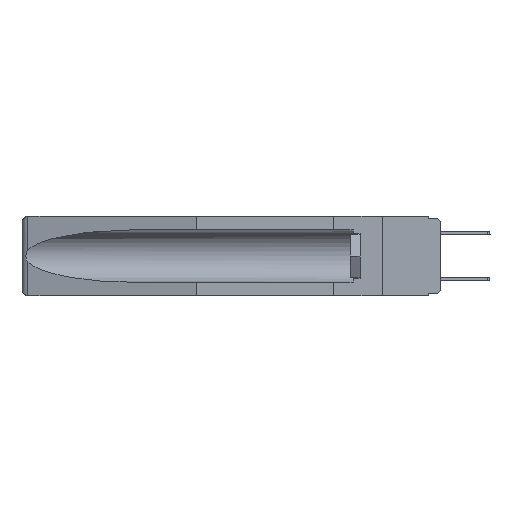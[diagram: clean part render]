
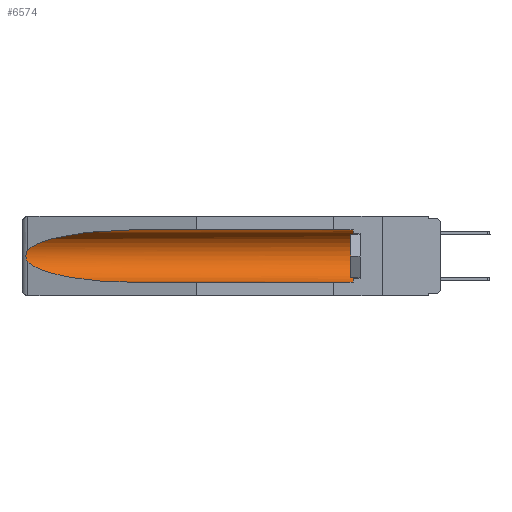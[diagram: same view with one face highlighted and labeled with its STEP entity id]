
A CAD part, left-side view. The second image highlights one B-rep face of the part: STEP entity #6574.
In plain terms, the highlighted cylindrical face has radius 2.857 mm (diameter 5.715 mm), a partial arc.
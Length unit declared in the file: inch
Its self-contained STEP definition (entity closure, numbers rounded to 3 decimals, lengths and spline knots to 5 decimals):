
#9 = CARTESIAN_POINT ( 'NONE',  ( 0.2675, 1.53308, -0.17534 ) ) ;
#93 =( BOUNDED_CURVE ( )  B_SPLINE_CURVE ( 3, ( #5002, #11136, #8118, #14259 ),
 .UNSPECIFIED., .F., .F. ) 
 B_SPLINE_CURVE_WITH_KNOTS ( ( 4, 4 ),
 ( 0.1948, 1.5708 ),
 .UNSPECIFIED. ) 
 CURVE ( )  GEOMETRIC_REPRESENTATION_ITEM ( )  RATIONAL_B_SPLINE_CURVE ( ( 1., 0.848, 0.848, 1. ) ) 
 REPRESENTATION_ITEM ( '' )  );
#108 = FACE_OUTER_BOUND ( 'NONE', #941, .T. ) ;
#810 = CARTESIAN_POINT ( 'NONE',  ( 0.26537, 1.52718, -0.14972 ) ) ;
#941 = EDGE_LOOP ( 'NONE', ( #19492, #7121, #16812, #2679, #1300, #1468 ) ) ;
#1225 = CARTESIAN_POINT ( 'NONE',  ( 0.26597, 1.52961, -0.15275 ) ) ;
#1300 = ORIENTED_EDGE ( 'NONE', *, *, #8733, .T. ) ;
#1468 = ORIENTED_EDGE ( 'NONE', *, *, #6871, .T. ) ;
#1628 = CARTESIAN_POINT ( 'NONE',  ( 0.26537, 1.52718, -0.14972 ) ) ;
#1767 = VERTEX_POINT ( 'NONE', #19756 ) ;
#2050 = CARTESIAN_POINT ( 'NONE',  ( 0.155, 0.126, -0.284 ) ) ;
#2679 = ORIENTED_EDGE ( 'NONE', *, *, #15390, .F. ) ;
#2933 = CARTESIAN_POINT ( 'NONE',  ( 0.26597, 1.5296, -0.19026 ) ) ;
#3026 = LINE ( 'NONE', #10571, #8775 ) ;
#3757 = CARTESIAN_POINT ( 'NONE',  ( 0.26537, 1.52718, -0.19328 ) ) ;
#3776 = AXIS2_PLACEMENT_3D ( 'NONE', #12192, #8975, #9161 ) ;
#4337 = CARTESIAN_POINT ( 'NONE',  ( 0.26537, 1.52718, -0.19328 ) ) ;
#4497 = DIRECTION ( 'NONE',  ( 0., 0., 1. ) ) ;
#5002 = CARTESIAN_POINT ( 'NONE',  ( 0.26537, 1.52718, -0.19328 ) ) ;
#5300 = EDGE_CURVE ( 'NONE', #17446, #18769, #6170, .T. ) ;
#5739 = AXIS2_PLACEMENT_3D ( 'NONE', #15371, #19775, #4497 ) ;
#6170 = B_SPLINE_CURVE_WITH_KNOTS ( 'NONE', 3,
 ( #1628, #1225, #10573, #18117, #19816, #9, #12291, #7372, #2933, #4337 ),
 .UNSPECIFIED., .F., .F.,
 ( 4, 2, 2, 2, 4 ),
 ( 0., 0.00029, 0.00058, 0.00087, 0.00117 ),
 .UNSPECIFIED. ) ;
#6574 = ADVANCED_FACE ( 'NONE', ( #108 ), #7859, .F. ) ;
#6871 = EDGE_CURVE ( 'NONE', #15940, #9825, #19199, .T. ) ;
#6949 = DIRECTION ( 'NONE',  ( 0., 1., 0. ) ) ;
#7121 = ORIENTED_EDGE ( 'NONE', *, *, #5300, .T. ) ;
#7372 = CARTESIAN_POINT ( 'NONE',  ( 0.26655, 1.53094, -0.18657 ) ) ;
#7859 = CYLINDRICAL_SURFACE ( 'NONE', #3776, 0.1125 ) ;
#8118 = CARTESIAN_POINT ( 'NONE',  ( 0.21114, 1.30732, -0.284 ) ) ;
#8733 = EDGE_CURVE ( 'NONE', #12511, #15940, #9894, .T. ) ;
#8775 = VECTOR ( 'NONE', #8867, 39.37008 ) ;
#8867 = DIRECTION ( 'NONE',  ( 0., 1., 0. ) ) ;
#8975 = DIRECTION ( 'NONE',  ( 0., 1., 0. ) ) ;
#9161 = DIRECTION ( 'NONE',  ( 0., 0., 1. ) ) ;
#9825 = VERTEX_POINT ( 'NONE', #13916 ) ;
#9894 = CIRCLE ( 'NONE', #5739, 0.1125 ) ;
#10571 = CARTESIAN_POINT ( 'NONE',  ( 0.155, -0.30754, -0.284 ) ) ;
#10573 = CARTESIAN_POINT ( 'NONE',  ( 0.26654, 1.53092, -0.15636 ) ) ;
#11136 = CARTESIAN_POINT ( 'NONE',  ( 0.25451, 1.48313, -0.24835 ) ) ;
#11821 = VECTOR ( 'NONE', #6949, 39.37008 ) ;
#12000 = EDGE_CURVE ( 'NONE', #18769, #1767, #93, .T. ) ;
#12192 = CARTESIAN_POINT ( 'NONE',  ( 0.155, -0.30754, -0.1715 ) ) ;
#12291 = CARTESIAN_POINT ( 'NONE',  ( 0.2673, 1.53269, -0.17917 ) ) ;
#12511 = VERTEX_POINT ( 'NONE', #2050 ) ;
#12665 = CARTESIAN_POINT ( 'NONE',  ( 0.155, 0.126, -0.059 ) ) ;
#13099 = EDGE_CURVE ( 'NONE', #9825, #17446, #15804, .T. ) ;
#13573 = CARTESIAN_POINT ( 'NONE',  ( 0.26537, 1.52718, -0.14972 ) ) ;
#13768 = CARTESIAN_POINT ( 'NONE',  ( 0.25451, 1.48313, -0.09465 ) ) ;
#13916 = CARTESIAN_POINT ( 'NONE',  ( 0.155, 1.07973, -0.059 ) ) ;
#14259 = CARTESIAN_POINT ( 'NONE',  ( 0.155, 1.07973, -0.284 ) ) ;
#14980 = CARTESIAN_POINT ( 'NONE',  ( 0.155, 1.07973, -0.059 ) ) ;
#15371 = CARTESIAN_POINT ( 'NONE',  ( 0.155, 0.126, -0.1715 ) ) ;
#15390 = EDGE_CURVE ( 'NONE', #12511, #1767, #3026, .T. ) ;
#15804 =( BOUNDED_CURVE ( )  B_SPLINE_CURVE ( 3, ( #14980, #16575, #13768, #13573 ),
 .UNSPECIFIED., .F., .F. ) 
 B_SPLINE_CURVE_WITH_KNOTS ( ( 4, 4 ),
 ( 4.71239, 6.08839 ),
 .UNSPECIFIED. ) 
 CURVE ( )  GEOMETRIC_REPRESENTATION_ITEM ( )  RATIONAL_B_SPLINE_CURVE ( ( 1., 0.848, 0.848, 1. ) ) 
 REPRESENTATION_ITEM ( '' )  );
#15940 = VERTEX_POINT ( 'NONE', #12665 ) ;
#16103 = CARTESIAN_POINT ( 'NONE',  ( 0.155, -0.30754, -0.059 ) ) ;
#16575 = CARTESIAN_POINT ( 'NONE',  ( 0.21114, 1.30732, -0.059 ) ) ;
#16812 = ORIENTED_EDGE ( 'NONE', *, *, #12000, .T. ) ;
#17446 = VERTEX_POINT ( 'NONE', #810 ) ;
#18117 = CARTESIAN_POINT ( 'NONE',  ( 0.2673, 1.5327, -0.16383 ) ) ;
#18769 = VERTEX_POINT ( 'NONE', #3757 ) ;
#19199 = LINE ( 'NONE', #16103, #11821 ) ;
#19492 = ORIENTED_EDGE ( 'NONE', *, *, #13099, .T. ) ;
#19756 = CARTESIAN_POINT ( 'NONE',  ( 0.155, 1.07973, -0.284 ) ) ;
#19775 = DIRECTION ( 'NONE',  ( 0., -1., 0. ) ) ;
#19816 = CARTESIAN_POINT ( 'NONE',  ( 0.2675, 1.53308, -0.16763 ) ) ;
